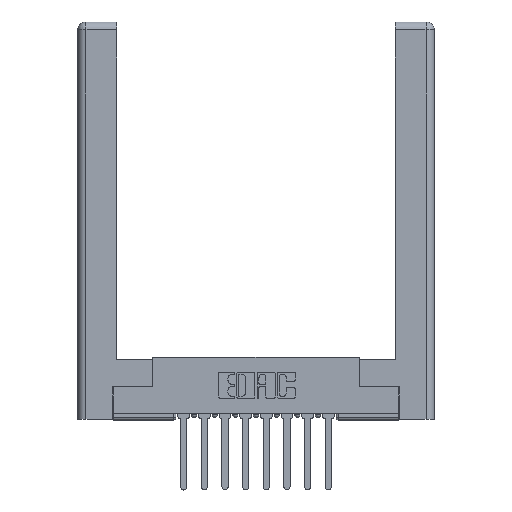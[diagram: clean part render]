
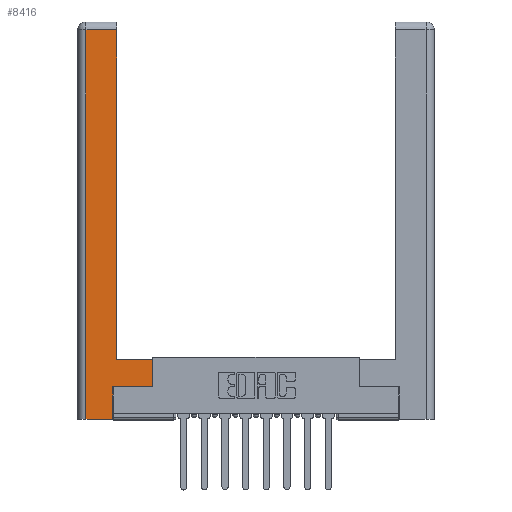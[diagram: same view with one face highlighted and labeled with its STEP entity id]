
A CAD part, top view. The second image highlights one B-rep face of the part: STEP entity #8416.
In plain terms, the highlighted planar face has unit normal (0, 0, 1).
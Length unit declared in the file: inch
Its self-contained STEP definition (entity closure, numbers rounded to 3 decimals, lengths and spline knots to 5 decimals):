
#43 = ORIENTED_EDGE ( 'NONE', *, *, #3662, .T. ) ;
#88 = CARTESIAN_POINT ( 'NONE',  ( 0.565, 0.45, 0. ) ) ;
#182 = FACE_OUTER_BOUND ( 'NONE', #7916, .T. ) ;
#385 = CARTESIAN_POINT ( 'NONE',  ( 0.265, 0., 0. ) ) ;
#599 = CARTESIAN_POINT ( 'NONE',  ( 0.565, 0.245, 0. ) ) ;
#832 = DIRECTION ( 'NONE',  ( -1., 0., 0. ) ) ;
#904 = CARTESIAN_POINT ( 'NONE',  ( 0.0615, 0., 0. ) ) ;
#949 = LINE ( 'NONE', #88, #5570 ) ;
#1308 = VECTOR ( 'NONE', #8902, 39.37008 ) ;
#1450 = DIRECTION ( 'NONE',  ( 1., 0., 0. ) ) ;
#1693 = VERTEX_POINT ( 'NONE', #8954 ) ;
#2120 = ORIENTED_EDGE ( 'NONE', *, *, #7152, .T. ) ;
#2303 = LINE ( 'NONE', #385, #10563 ) ;
#2646 = AXIS2_PLACEMENT_3D ( 'NONE', #3836, #10229, #832 ) ;
#2783 = PLANE ( 'NONE',  #2646 ) ;
#2909 = CARTESIAN_POINT ( 'NONE',  ( 0.265, 0.245, 0. ) ) ;
#3111 = VERTEX_POINT ( 'NONE', #10354 ) ;
#3191 = LINE ( 'NONE', #6667, #11456 ) ;
#3517 = ORIENTED_EDGE ( 'NONE', *, *, #6357, .T. ) ;
#3662 = EDGE_CURVE ( 'NONE', #10933, #13073, #3191, .T. ) ;
#3665 = LINE ( 'NONE', #2909, #11748 ) ;
#3675 = EDGE_CURVE ( 'NONE', #3111, #10933, #8161, .T. ) ;
#3688 = VECTOR ( 'NONE', #4607, 39.37008 ) ;
#3813 = DIRECTION ( 'NONE',  ( 1., 0., 0. ) ) ;
#3836 = CARTESIAN_POINT ( 'NONE',  ( 0., 0., 0. ) ) ;
#3872 = ORIENTED_EDGE ( 'NONE', *, *, #10000, .T. ) ;
#3918 = LINE ( 'NONE', #599, #4084 ) ;
#4084 = VECTOR ( 'NONE', #3813, 39.37008 ) ;
#4607 = DIRECTION ( 'NONE',  ( 0., 1., 0. ) ) ;
#5447 = EDGE_CURVE ( 'NONE', #13073, #6526, #13190, .T. ) ;
#5570 = VECTOR ( 'NONE', #6475, 39.37008 ) ;
#5734 = ORIENTED_EDGE ( 'NONE', *, *, #10306, .T. ) ;
#5984 = CARTESIAN_POINT ( 'NONE',  ( 0.565, 0.245, 0. ) ) ;
#6340 = EDGE_CURVE ( 'NONE', #6963, #3111, #12681, .T. ) ;
#6357 = EDGE_CURVE ( 'NONE', #6526, #12032, #2303, .T. ) ;
#6462 = CARTESIAN_POINT ( 'NONE',  ( 0.295, 2.94, 0. ) ) ;
#6475 = DIRECTION ( 'NONE',  ( 0., 1., 0. ) ) ;
#6526 = VERTEX_POINT ( 'NONE', #9445 ) ;
#6667 = CARTESIAN_POINT ( 'NONE',  ( 0.0615, 2.94, 0. ) ) ;
#6910 = CARTESIAN_POINT ( 'NONE',  ( 0.565, 0.45, 0. ) ) ;
#6963 = VERTEX_POINT ( 'NONE', #6910 ) ;
#7152 = EDGE_CURVE ( 'NONE', #12032, #1693, #3665, .T. ) ;
#7303 = DIRECTION ( 'NONE',  ( 0., -1., 0. ) ) ;
#7916 = EDGE_LOOP ( 'NONE', ( #11148, #43, #12963, #3517, #2120, #3872, #5734, #9263 ) ) ;
#8161 = LINE ( 'NONE', #10904, #3688 ) ;
#8416 = ADVANCED_FACE ( 'NONE', ( #182 ), #2783, .F. ) ;
#8445 = CARTESIAN_POINT ( 'NONE',  ( 0.0615, 2.94, 0. ) ) ;
#8902 = DIRECTION ( 'NONE',  ( -1., 0., 0. ) ) ;
#8954 = CARTESIAN_POINT ( 'NONE',  ( 0.265, 0.245, 0. ) ) ;
#9263 = ORIENTED_EDGE ( 'NONE', *, *, #6340, .T. ) ;
#9281 = VERTEX_POINT ( 'NONE', #5984 ) ;
#9445 = CARTESIAN_POINT ( 'NONE',  ( 0.0615, 0., 0. ) ) ;
#9592 = CARTESIAN_POINT ( 'NONE',  ( 0.265, 0., 0. ) ) ;
#10000 = EDGE_CURVE ( 'NONE', #1693, #9281, #3918, .T. ) ;
#10229 = DIRECTION ( 'NONE',  ( 0., 0., -1. ) ) ;
#10306 = EDGE_CURVE ( 'NONE', #9281, #6963, #949, .T. ) ;
#10354 = CARTESIAN_POINT ( 'NONE',  ( 0.295, 0.45, 0. ) ) ;
#10563 = VECTOR ( 'NONE', #1450, 39.37008 ) ;
#10904 = CARTESIAN_POINT ( 'NONE',  ( 0.295, 3., 0. ) ) ;
#10933 = VERTEX_POINT ( 'NONE', #6462 ) ;
#11148 = ORIENTED_EDGE ( 'NONE', *, *, #3675, .T. ) ;
#11456 = VECTOR ( 'NONE', #12906, 39.37008 ) ;
#11718 = VECTOR ( 'NONE', #7303, 39.37008 ) ;
#11748 = VECTOR ( 'NONE', #13510, 39.37008 ) ;
#12032 = VERTEX_POINT ( 'NONE', #9592 ) ;
#12681 = LINE ( 'NONE', #13011, #1308 ) ;
#12906 = DIRECTION ( 'NONE',  ( -1., 0., 0. ) ) ;
#12963 = ORIENTED_EDGE ( 'NONE', *, *, #5447, .T. ) ;
#13011 = CARTESIAN_POINT ( 'NONE',  ( 0.295, 0.45, 0. ) ) ;
#13073 = VERTEX_POINT ( 'NONE', #8445 ) ;
#13190 = LINE ( 'NONE', #904, #11718 ) ;
#13510 = DIRECTION ( 'NONE',  ( 0., 1., 0. ) ) ;
